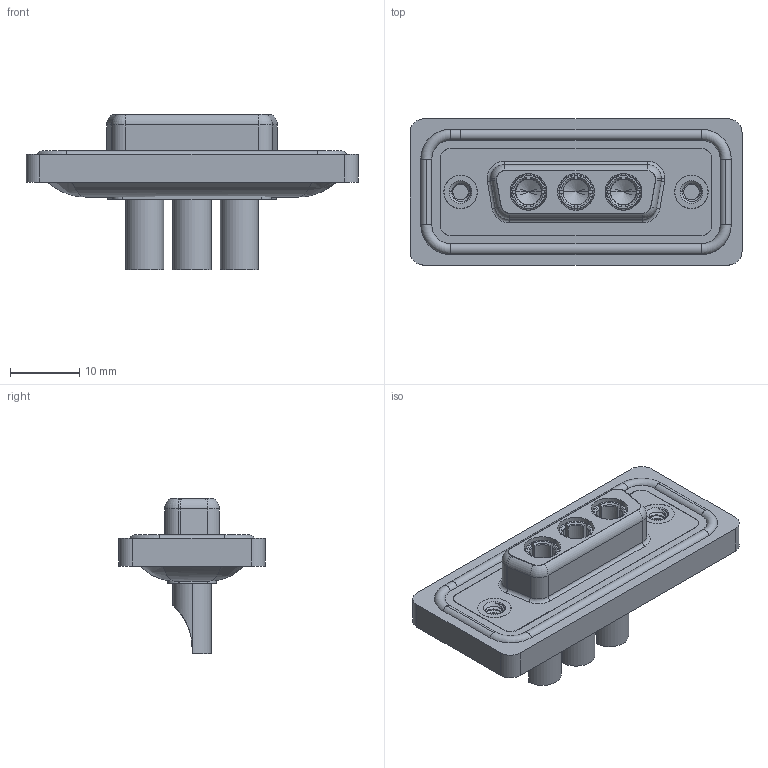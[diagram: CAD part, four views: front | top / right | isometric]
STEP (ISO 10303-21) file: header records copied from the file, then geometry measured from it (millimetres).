
FILE_DESCRIPTION (( 'STEP AP203' ), '1' );
FILE_NAME ('628W3W3-122-4N2.STEP', '2024-03-22T14:32:36', ( '' ), ( '' ), 'SwSTEP 2.0', 'SolidWorks 2023', '' );
FILE_SCHEMA (( 'CONFIG_CONTROL_DESIGN' ));
Length unit declared in the file: millimetre
Products named in the file (7): 628W3W3-122-4N2; 628Combo Threaded Rivet_2; 628Combo Shell Front_15 Contacts; Power Socket_40A SC; 628Combo Housing_3W3; 628Combo Shell Rear_15 Contacts; 628Combo Waterproof Housing_15 Contacts
Assembly tree (9 placements, depth 2):
  628W3W3-122-4N2
    628Combo Housing_3W3
    628Combo Waterproof Housing_15 Contacts
    628Combo Shell Front_15 Contacts
    628Combo Shell Rear_15 Contacts
    628Combo Threaded Rivet_2  x2
    Power Socket_40A SC  x3
Bounding box: 47.9 x 21.1 x 22.45 mm (x, y, z)
Volume: 6146.1 mm3; surface area: 10158.2 mm2
Topology: 13 solids, 13 shells, 617 faces, 1578 edges, 994 vertices
Faces by surface type: cylinder 260, plane 198, torus 83, cone 63, bspline 13
Entity records: 15994 total; most frequent: CARTESIAN_POINT 4537, DIRECTION 2333, ORIENTED_EDGE 2194, EDGE_CURVE 1097, AXIS2_PLACEMENT_3D 929, VERTEX_POINT 694, CIRCLE 485, EDGE_LOOP 483
